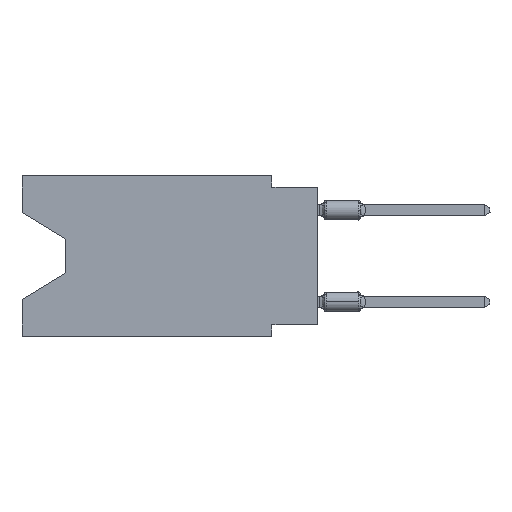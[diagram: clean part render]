
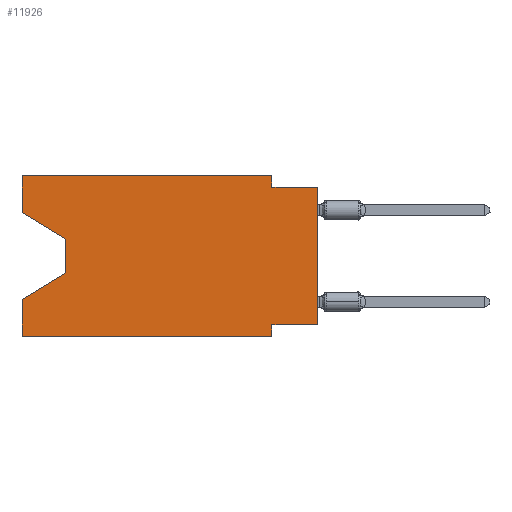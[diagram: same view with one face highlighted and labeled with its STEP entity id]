
A CAD part, left-side view. The second image highlights one B-rep face of the part: STEP entity #11926.
In plain terms, the highlighted planar face has unit normal (-1, 0, 0).
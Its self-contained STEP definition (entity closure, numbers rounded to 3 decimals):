
#443 = LINE ( 'NONE', #49976, #8964 ) ;
#1148 = VERTEX_POINT ( 'NONE', #30609 ) ;
#1735 = CARTESIAN_POINT ( 'NONE',  ( 0., 16.383, -2.038 ) ) ;
#2094 = ORIENTED_EDGE ( 'NONE', *, *, #6084, .F. ) ;
#3887 = VERTEX_POINT ( 'NONE', #35384 ) ;
#4051 = EDGE_CURVE ( 'NONE', #61913, #1148, #42842, .T. ) ;
#4367 = CARTESIAN_POINT ( 'NONE',  ( 0., 16.383, 0. ) ) ;
#4905 = VERTEX_POINT ( 'NONE', #40408 ) ;
#5495 = VERTEX_POINT ( 'NONE', #24293 ) ;
#6077 = FACE_OUTER_BOUND ( 'NONE', #21942, .T. ) ;
#6084 = EDGE_CURVE ( 'NONE', #61913, #3887, #37990, .T. ) ;
#6458 = ORIENTED_EDGE ( 'NONE', *, *, #59976, .F. ) ;
#7580 = DIRECTION ( 'NONE',  ( 0., -0.855, -0.519 ) ) ;
#8095 = EDGE_CURVE ( 'NONE', #46634, #4905, #52265, .T. ) ;
#8292 = VERTEX_POINT ( 'NONE', #1735 ) ;
#8361 = LINE ( 'NONE', #24399, #40680 ) ;
#8964 = VECTOR ( 'NONE', #65687, 1000. ) ;
#10383 = DIRECTION ( 'NONE',  ( 1., 0., 0. ) ) ;
#10763 = LINE ( 'NONE', #49585, #38017 ) ;
#11926 = ADVANCED_FACE ( 'NONE', ( #6077 ), #27812, .F. ) ;
#11982 = DIRECTION ( 'NONE',  ( 0., 0., 1. ) ) ;
#12720 = CARTESIAN_POINT ( 'NONE',  ( 0., 13.97, -3.505 ) ) ;
#14901 = EDGE_CURVE ( 'NONE', #40978, #5495, #8361, .T. ) ;
#15411 = DIRECTION ( 'NONE',  ( 0., -1., 0. ) ) ;
#15754 = VECTOR ( 'NONE', #41916, 1000. ) ;
#16513 = ORIENTED_EDGE ( 'NONE', *, *, #31765, .T. ) ;
#16775 = DIRECTION ( 'NONE',  ( 0., 0., -1. ) ) ;
#16811 = CARTESIAN_POINT ( 'NONE',  ( 0., 16.383, -8.89 ) ) ;
#18037 = LINE ( 'NONE', #50808, #56551 ) ;
#18102 = EDGE_CURVE ( 'NONE', #5495, #1148, #443, .T. ) ;
#18472 = ORIENTED_EDGE ( 'NONE', *, *, #26473, .T. ) ;
#20173 = CARTESIAN_POINT ( 'NONE',  ( 0., 0., -0.635 ) ) ;
#20311 = DIRECTION ( 'NONE',  ( 0., -1., 0. ) ) ;
#21942 = EDGE_LOOP ( 'NONE', ( #64309, #18472, #69116, #2094, #25776, #65561, #47643, #16513, #37844, #6458, #49632, #49296 ) ) ;
#22952 = CARTESIAN_POINT ( 'NONE',  ( 0., 13.97, -3.505 ) ) ;
#24293 = CARTESIAN_POINT ( 'NONE',  ( 0., 2.54, -8.255 ) ) ;
#24331 = CARTESIAN_POINT ( 'NONE',  ( 0., 13.97, -5.385 ) ) ;
#24399 = CARTESIAN_POINT ( 'NONE',  ( 0., 0., -8.255 ) ) ;
#25035 = AXIS2_PLACEMENT_3D ( 'NONE', #27466, #10383, #16775 ) ;
#25038 = LINE ( 'NONE', #68554, #29274 ) ;
#25776 = ORIENTED_EDGE ( 'NONE', *, *, #4051, .T. ) ;
#26473 = EDGE_CURVE ( 'NONE', #37333, #62053, #61550, .T. ) ;
#26480 = CARTESIAN_POINT ( 'NONE',  ( 0., 0., 0. ) ) ;
#27466 = CARTESIAN_POINT ( 'NONE',  ( 0., 16.383, 0. ) ) ;
#27812 = PLANE ( 'NONE',  #25035 ) ;
#28957 = VERTEX_POINT ( 'NONE', #55438 ) ;
#29274 = VECTOR ( 'NONE', #7580, 1000. ) ;
#30370 = DIRECTION ( 'NONE',  ( 0., 0.855, -0.519 ) ) ;
#30609 = CARTESIAN_POINT ( 'NONE',  ( 0., 2.54, -8.89 ) ) ;
#31147 = VECTOR ( 'NONE', #15411, 1000. ) ;
#31765 = EDGE_CURVE ( 'NONE', #40978, #4905, #43233, .T. ) ;
#32529 = DIRECTION ( 'NONE',  ( 0., 0., 1. ) ) ;
#33513 = CARTESIAN_POINT ( 'NONE',  ( 0., 16.383, -8.89 ) ) ;
#35384 = CARTESIAN_POINT ( 'NONE',  ( 0., 16.383, -6.852 ) ) ;
#35452 = VECTOR ( 'NONE', #32529, 1000. ) ;
#35991 = LINE ( 'NONE', #42759, #58484 ) ;
#37333 = VERTEX_POINT ( 'NONE', #22952 ) ;
#37844 = ORIENTED_EDGE ( 'NONE', *, *, #8095, .F. ) ;
#37990 = LINE ( 'NONE', #59735, #62197 ) ;
#38017 = VECTOR ( 'NONE', #54243, 1000. ) ;
#40408 = CARTESIAN_POINT ( 'NONE',  ( 0., 0., -0.635 ) ) ;
#40680 = VECTOR ( 'NONE', #52905, 1000. ) ;
#40723 = LINE ( 'NONE', #24331, #61891 ) ;
#40978 = VERTEX_POINT ( 'NONE', #51711 ) ;
#41304 = CARTESIAN_POINT ( 'NONE',  ( 0., 13.97, -5.385 ) ) ;
#41916 = DIRECTION ( 'NONE',  ( 0., -1., 0. ) ) ;
#42309 = VERTEX_POINT ( 'NONE', #4367 ) ;
#42542 = EDGE_CURVE ( 'NONE', #8292, #42309, #18037, .T. ) ;
#42759 = CARTESIAN_POINT ( 'NONE',  ( 0., 16.383, 0. ) ) ;
#42842 = LINE ( 'NONE', #16811, #31147 ) ;
#43233 = LINE ( 'NONE', #26480, #35452 ) ;
#43275 = EDGE_CURVE ( 'NONE', #8292, #37333, #25038, .T. ) ;
#46634 = VERTEX_POINT ( 'NONE', #57146 ) ;
#47643 = ORIENTED_EDGE ( 'NONE', *, *, #14901, .F. ) ;
#49296 = ORIENTED_EDGE ( 'NONE', *, *, #42542, .F. ) ;
#49583 = VECTOR ( 'NONE', #68660, 1000. ) ;
#49585 = CARTESIAN_POINT ( 'NONE',  ( 0., 2.54, 0. ) ) ;
#49632 = ORIENTED_EDGE ( 'NONE', *, *, #60267, .F. ) ;
#49976 = CARTESIAN_POINT ( 'NONE',  ( 0., 2.54, -8.89 ) ) ;
#50808 = CARTESIAN_POINT ( 'NONE',  ( 0., 16.383, 0. ) ) ;
#51711 = CARTESIAN_POINT ( 'NONE',  ( 0., 0., -8.255 ) ) ;
#52265 = LINE ( 'NONE', #20173, #15754 ) ;
#52905 = DIRECTION ( 'NONE',  ( 0., 1., 0. ) ) ;
#54243 = DIRECTION ( 'NONE',  ( 0., 0., -1. ) ) ;
#54386 = DIRECTION ( 'NONE',  ( 0., 0., 1. ) ) ;
#55438 = CARTESIAN_POINT ( 'NONE',  ( 0., 2.54, 0. ) ) ;
#56551 = VECTOR ( 'NONE', #11982, 1000. ) ;
#57146 = CARTESIAN_POINT ( 'NONE',  ( 0., 2.54, -0.635 ) ) ;
#58484 = VECTOR ( 'NONE', #20311, 1000. ) ;
#59692 = EDGE_CURVE ( 'NONE', #62053, #3887, #40723, .T. ) ;
#59735 = CARTESIAN_POINT ( 'NONE',  ( 0., 16.383, 0. ) ) ;
#59976 = EDGE_CURVE ( 'NONE', #28957, #46634, #10763, .T. ) ;
#60267 = EDGE_CURVE ( 'NONE', #42309, #28957, #35991, .T. ) ;
#61550 = LINE ( 'NONE', #12720, #49583 ) ;
#61891 = VECTOR ( 'NONE', #30370, 1000. ) ;
#61913 = VERTEX_POINT ( 'NONE', #33513 ) ;
#62053 = VERTEX_POINT ( 'NONE', #41304 ) ;
#62197 = VECTOR ( 'NONE', #54386, 1000. ) ;
#64309 = ORIENTED_EDGE ( 'NONE', *, *, #43275, .T. ) ;
#65561 = ORIENTED_EDGE ( 'NONE', *, *, #18102, .F. ) ;
#65687 = DIRECTION ( 'NONE',  ( 0., 0., -1. ) ) ;
#68554 = CARTESIAN_POINT ( 'NONE',  ( 0., 16.383, -2.038 ) ) ;
#68660 = DIRECTION ( 'NONE',  ( 0., 0., -1. ) ) ;
#69116 = ORIENTED_EDGE ( 'NONE', *, *, #59692, .T. ) ;
